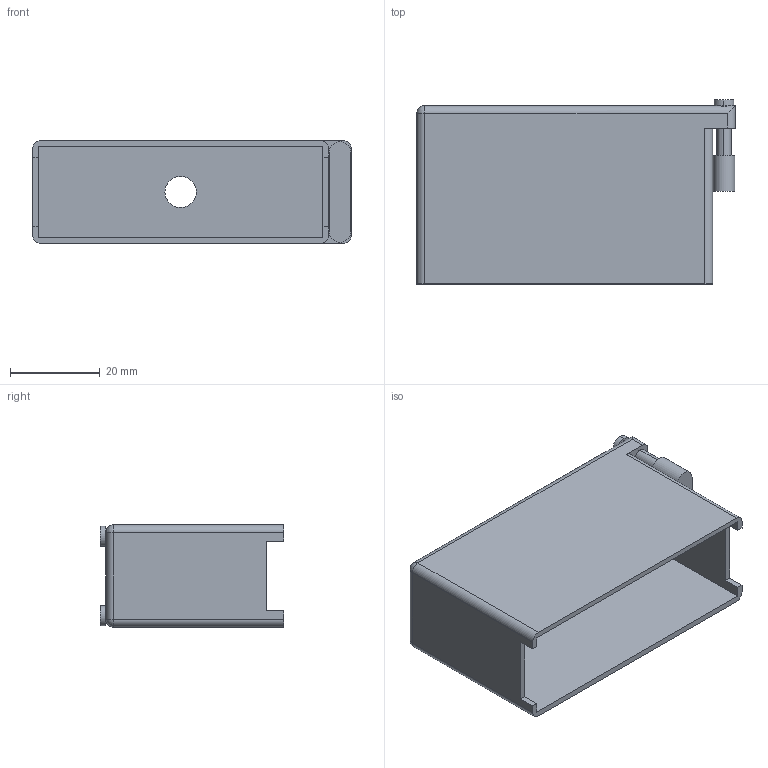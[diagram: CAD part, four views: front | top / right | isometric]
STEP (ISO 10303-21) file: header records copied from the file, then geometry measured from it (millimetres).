
FILE_DESCRIPTION (( 'STEP AP214' ), '1' );
FILE_NAME ('516-230-556.STEP', '2020-08-14T15:38:53', ( '' ), ( '' ), 'SwSTEP 2.0', 'SolidWorks 2020', '' );
FILE_SCHEMA (( 'AUTOMOTIVE_DESIGN' ));
Length unit declared in the file: millimetre
Products named in the file (2): 516-230-556; 516-230-001_Metal - 056 Side Entry
Assembly tree (1 placements, depth 2):
  516-230-556
    516-230-001_Metal - 056 Side Entry
Bounding box: 71.12 x 41.05 x 22.83 mm (x, y, z)
Volume: 10675.6 mm3; surface area: 16529.4 mm2
Topology: 1 solids, 1 shells, 62 faces, 167 edges, 106 vertices
Faces by surface type: plane 33, cylinder 27, sphere 2
Entity records: 2141 total; most frequent: CARTESIAN_POINT 378, DIRECTION 343, ORIENTED_EDGE 330, EDGE_CURVE 165, AXIS2_PLACEMENT_3D 117, LINE 109, VECTOR 109, VERTEX_POINT 106
